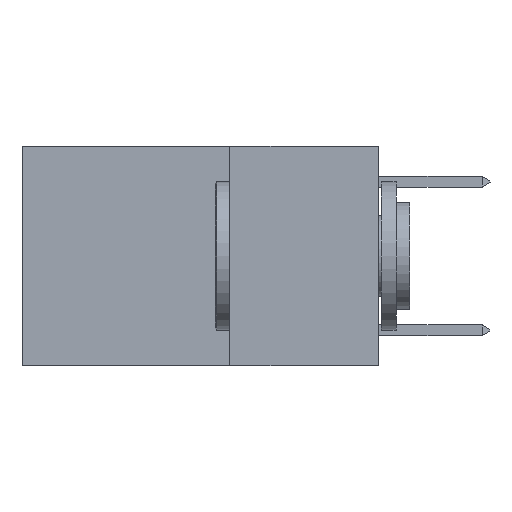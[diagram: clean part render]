
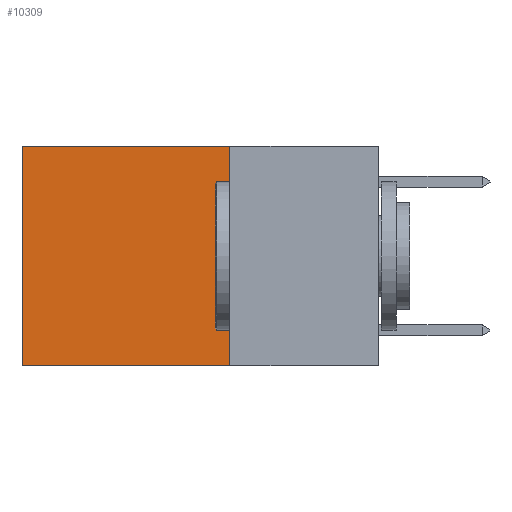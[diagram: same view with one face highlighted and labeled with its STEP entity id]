
A CAD part, left-side view. The second image highlights one B-rep face of the part: STEP entity #10309.
In plain terms, the highlighted planar face has unit normal (-1, 0, 0).
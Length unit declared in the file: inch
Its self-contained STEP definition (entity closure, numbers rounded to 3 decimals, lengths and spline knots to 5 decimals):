
#184 = AXIS2_PLACEMENT_3D ( 'NONE', #4411, #5307, #6038 ) ;
#257 = PLANE ( 'NONE',  #184 ) ;
#466 = FACE_OUTER_BOUND ( 'NONE', #470, .T. ) ;
#470 = EDGE_LOOP ( 'NONE', ( #8546, #2320, #9415, #2282 ) ) ;
#644 = DIRECTION ( 'NONE',  ( 0., 0., -1. ) ) ;
#661 = VECTOR ( 'NONE', #885, 39.37008 ) ;
#722 = CARTESIAN_POINT ( 'NONE',  ( 0.2625, 0.25, 0. ) ) ;
#832 = CARTESIAN_POINT ( 'NONE',  ( 0.2625, 0.6, -0.37 ) ) ;
#885 = DIRECTION ( 'NONE',  ( 0., 1., 0. ) ) ;
#1285 = LINE ( 'NONE', #6750, #2175 ) ;
#1343 = EDGE_CURVE ( 'NONE', #3575, #9317, #1285, .T. ) ;
#1381 = VERTEX_POINT ( 'NONE', #6972 ) ;
#2175 = VECTOR ( 'NONE', #5166, 39.37008 ) ;
#2281 = EDGE_CURVE ( 'NONE', #3575, #1381, #10478, .T. ) ;
#2282 = ORIENTED_EDGE ( 'NONE', *, *, #2281, .T. ) ;
#2320 = ORIENTED_EDGE ( 'NONE', *, *, #3613, .F. ) ;
#2349 = CARTESIAN_POINT ( 'NONE',  ( 0.2625, 0.6, 0. ) ) ;
#3105 = CARTESIAN_POINT ( 'NONE',  ( 0.2625, 0.25, 0. ) ) ;
#3575 = VERTEX_POINT ( 'NONE', #3105 ) ;
#3613 = EDGE_CURVE ( 'NONE', #9317, #4606, #6174, .T. ) ;
#3649 = CARTESIAN_POINT ( 'NONE',  ( 0.2625, 0.25, -0.37 ) ) ;
#4411 = CARTESIAN_POINT ( 'NONE',  ( 0.2625, 0.25, 0. ) ) ;
#4598 = CARTESIAN_POINT ( 'NONE',  ( 0.2625, 0.25, -0.37 ) ) ;
#4606 = VERTEX_POINT ( 'NONE', #832 ) ;
#5166 = DIRECTION ( 'NONE',  ( 0., 0., -1. ) ) ;
#5307 = DIRECTION ( 'NONE',  ( 1., 0., 0. ) ) ;
#5915 = VECTOR ( 'NONE', #644, 39.37008 ) ;
#6038 = DIRECTION ( 'NONE',  ( 0., 0., -1. ) ) ;
#6174 = LINE ( 'NONE', #4598, #8149 ) ;
#6331 = DIRECTION ( 'NONE',  ( 0., 1., 0. ) ) ;
#6372 = LINE ( 'NONE', #2349, #5915 ) ;
#6703 = EDGE_CURVE ( 'NONE', #1381, #4606, #6372, .T. ) ;
#6750 = CARTESIAN_POINT ( 'NONE',  ( 0.2625, 0.25, 0. ) ) ;
#6972 = CARTESIAN_POINT ( 'NONE',  ( 0.2625, 0.6, 0. ) ) ;
#8149 = VECTOR ( 'NONE', #6331, 39.37008 ) ;
#8546 = ORIENTED_EDGE ( 'NONE', *, *, #6703, .T. ) ;
#9317 = VERTEX_POINT ( 'NONE', #3649 ) ;
#9415 = ORIENTED_EDGE ( 'NONE', *, *, #1343, .F. ) ;
#10309 = ADVANCED_FACE ( 'NONE', ( #466 ), #257, .F. ) ;
#10478 = LINE ( 'NONE', #722, #661 ) ;
